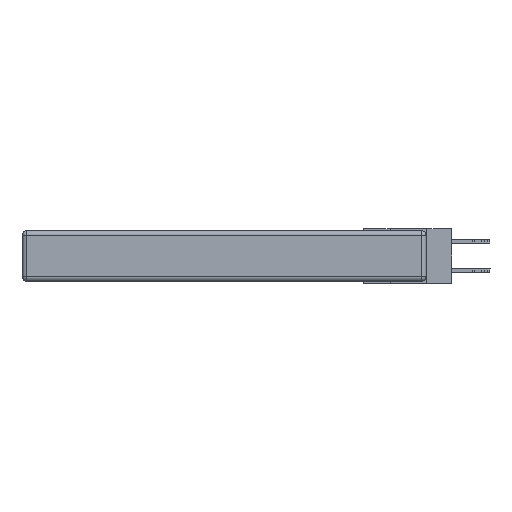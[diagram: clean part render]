
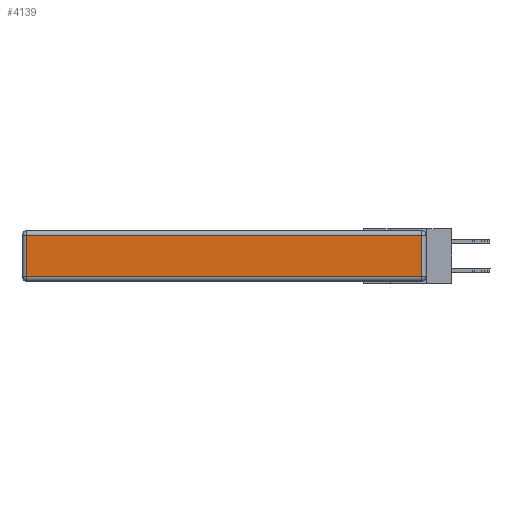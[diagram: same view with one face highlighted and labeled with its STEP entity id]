
A CAD part, left-side view. The second image highlights one B-rep face of the part: STEP entity #4139.
In plain terms, the highlighted planar face has unit normal (-1, 0, 0).
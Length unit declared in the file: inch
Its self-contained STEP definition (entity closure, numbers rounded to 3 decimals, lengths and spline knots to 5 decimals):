
#1755 = VECTOR ( 'NONE', #11383, 39.37008 ) ;
#2642 = LINE ( 'NONE', #28061, #1755 ) ;
#3180 = VERTEX_POINT ( 'NONE', #6853 ) ;
#3238 = DIRECTION ( 'NONE',  ( -1., 0., 0. ) ) ;
#4139 = ADVANCED_FACE ( 'NONE', ( #15406 ), #28435, .T. ) ;
#4159 = EDGE_LOOP ( 'NONE', ( #14685, #30547, #24719, #9764 ) ) ;
#5460 = VECTOR ( 'NONE', #17015, 39.37008 ) ;
#6853 = CARTESIAN_POINT ( 'NONE',  ( 0., 0.03, -0.313 ) ) ;
#6948 = VERTEX_POINT ( 'NONE', #23892 ) ;
#8463 = LINE ( 'NONE', #13990, #5460 ) ;
#9764 = ORIENTED_EDGE ( 'NONE', *, *, #32171, .T. ) ;
#11249 = CARTESIAN_POINT ( 'NONE',  ( 0., 0., -0.343 ) ) ;
#11383 = DIRECTION ( 'NONE',  ( 0., 0., 1. ) ) ;
#11548 = CARTESIAN_POINT ( 'NONE',  ( 0., 2.72, -0.313 ) ) ;
#12683 = VERTEX_POINT ( 'NONE', #35522 ) ;
#13990 = CARTESIAN_POINT ( 'NONE',  ( 0., 2.72, -0.343 ) ) ;
#14561 = EDGE_CURVE ( 'NONE', #29298, #3180, #17181, .T. ) ;
#14685 = ORIENTED_EDGE ( 'NONE', *, *, #14561, .T. ) ;
#15406 = FACE_OUTER_BOUND ( 'NONE', #4159, .T. ) ;
#15584 = DIRECTION ( 'NONE',  ( 0., -1., 0. ) ) ;
#17015 = DIRECTION ( 'NONE',  ( 0., 0., -1. ) ) ;
#17181 = LINE ( 'NONE', #27035, #31143 ) ;
#18284 = DIRECTION ( 'NONE',  ( 0., 1., 0. ) ) ;
#18535 = VECTOR ( 'NONE', #18284, 39.37008 ) ;
#19003 = LINE ( 'NONE', #26688, #18535 ) ;
#23892 = CARTESIAN_POINT ( 'NONE',  ( 0., 0.03, -0.03 ) ) ;
#24719 = ORIENTED_EDGE ( 'NONE', *, *, #31125, .T. ) ;
#25367 = DIRECTION ( 'NONE',  ( 0., 0., 1. ) ) ;
#26688 = CARTESIAN_POINT ( 'NONE',  ( 0., 2.75, -0.03 ) ) ;
#27035 = CARTESIAN_POINT ( 'NONE',  ( 0., 0., -0.313 ) ) ;
#27904 = AXIS2_PLACEMENT_3D ( 'NONE', #11249, #3238, #25367 ) ;
#28061 = CARTESIAN_POINT ( 'NONE',  ( 0., 0.03, -0.343 ) ) ;
#28435 = PLANE ( 'NONE',  #27904 ) ;
#29298 = VERTEX_POINT ( 'NONE', #11548 ) ;
#30547 = ORIENTED_EDGE ( 'NONE', *, *, #34247, .T. ) ;
#31125 = EDGE_CURVE ( 'NONE', #6948, #12683, #19003, .T. ) ;
#31143 = VECTOR ( 'NONE', #15584, 39.37008 ) ;
#32171 = EDGE_CURVE ( 'NONE', #12683, #29298, #8463, .T. ) ;
#34247 = EDGE_CURVE ( 'NONE', #3180, #6948, #2642, .T. ) ;
#35522 = CARTESIAN_POINT ( 'NONE',  ( 0., 2.72, -0.03 ) ) ;
